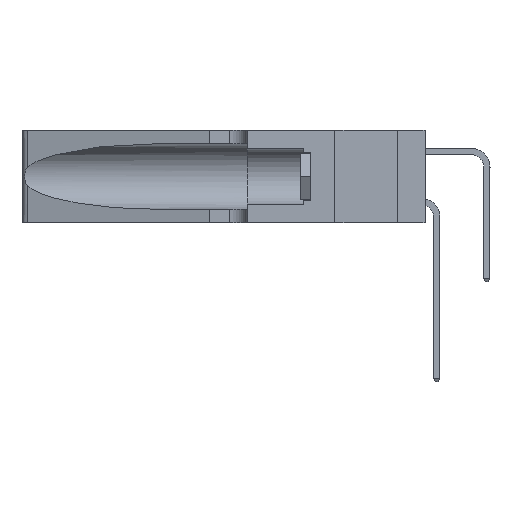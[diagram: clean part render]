
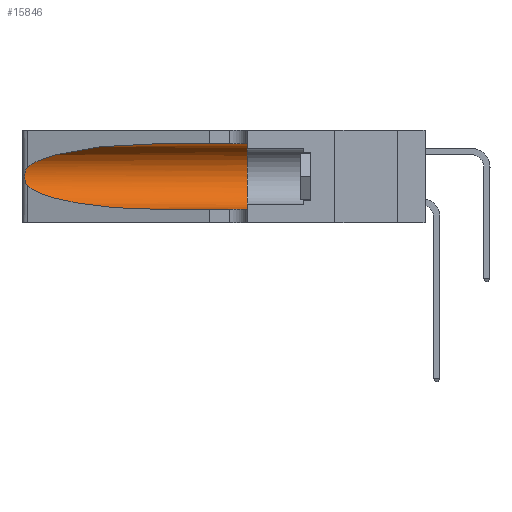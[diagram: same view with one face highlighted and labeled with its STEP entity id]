
A CAD part, left-side view. The second image highlights one B-rep face of the part: STEP entity #15846.
In plain terms, the highlighted cylindrical face has radius 3.308 mm (diameter 6.617 mm), a partial arc.
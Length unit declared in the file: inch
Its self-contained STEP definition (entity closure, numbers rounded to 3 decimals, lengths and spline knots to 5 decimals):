
#93 = CARTESIAN_POINT ( 'NONE',  ( 0.25487, 1.22718, 0.22369 ) ) ;
#305 = VERTEX_POINT ( 'NONE', #9422 ) ;
#831 = DIRECTION ( 'NONE',  ( 0., 1., 0. ) ) ;
#888 = ORIENTED_EDGE ( 'NONE', *, *, #11767, .T. ) ;
#2963 = DIRECTION ( 'NONE',  ( 0., -1., 0. ) ) ;
#3109 = CARTESIAN_POINT ( 'NONE',  ( 0.25487, 1.22718, 0.14631 ) ) ;
#3150 = FACE_OUTER_BOUND ( 'NONE', #14879, .T. ) ;
#3335 = VERTEX_POINT ( 'NONE', #10628 ) ;
#3477 = LINE ( 'NONE', #27125, #15596 ) ;
#3685 = CARTESIAN_POINT ( 'NONE',  ( 0.1305, 1.61858, 0.31525 ) ) ;
#3847 = CARTESIAN_POINT ( 'NONE',  ( 0.26018, 1.23835, 0.19895 ) ) ;
#4700 = DIRECTION ( 'NONE',  ( 0., 0., 1. ) ) ;
#5133 = AXIS2_PLACEMENT_3D ( 'NONE', #23783, #2963, #23971 ) ;
#5349 = VERTEX_POINT ( 'NONE', #10563 ) ;
#5922 = CARTESIAN_POINT ( 'NONE',  ( 0.25555, 1.22994, 0.2215 ) ) ;
#6010 = CARTESIAN_POINT ( 'NONE',  ( 0.25787, 1.23484, 0.2124 ) ) ;
#6208 = EDGE_CURVE ( 'NONE', #305, #3335, #11257, .T. ) ;
#6862 = ORIENTED_EDGE ( 'NONE', *, *, #12473, .F. ) ;
#7387 = CARTESIAN_POINT ( 'NONE',  ( 0.18966, 0.96281, 0.05475 ) ) ;
#8025 = CARTESIAN_POINT ( 'NONE',  ( 0.25856, 1.23593, 0.16098 ) ) ;
#8191 = CARTESIAN_POINT ( 'NONE',  ( 0.18966, 0.96281, 0.31525 ) ) ;
#8220 = LINE ( 'NONE', #3685, #18137 ) ;
#8479 = VERTEX_POINT ( 'NONE', #10007 ) ;
#9422 = CARTESIAN_POINT ( 'NONE',  ( 0.1305, 0.72297, 0.31525 ) ) ;
#10007 = CARTESIAN_POINT ( 'NONE',  ( 0.25487, 1.22718, 0.14631 ) ) ;
#10128 = CARTESIAN_POINT ( 'NONE',  ( 0.25639, 1.23186, 0.15144 ) ) ;
#10563 = CARTESIAN_POINT ( 'NONE',  ( 0.1305, 0.35, 0.31525 ) ) ;
#10628 = CARTESIAN_POINT ( 'NONE',  ( 0.25487, 1.22718, 0.22369 ) ) ;
#11150 = ORIENTED_EDGE ( 'NONE', *, *, #6208, .T. ) ;
#11257 =( BOUNDED_CURVE ( )  B_SPLINE_CURVE ( 3, ( #23757, #8191, #18303, #93 ),
 .UNSPECIFIED., .F., .T. ) 
 B_SPLINE_CURVE_WITH_KNOTS ( ( 4, 4 ),
 ( 1.5708, 2.84003 ),
 .UNSPECIFIED. ) 
 CURVE ( )  GEOMETRIC_REPRESENTATION_ITEM ( )  RATIONAL_B_SPLINE_CURVE ( ( 1., 0.87, 0.87, 1. ) ) 
 REPRESENTATION_ITEM ( '' )  );
#11392 = VERTEX_POINT ( 'NONE', #21391 ) ;
#11767 = EDGE_CURVE ( 'NONE', #8479, #15168, #16161, .T. ) ;
#12261 = CARTESIAN_POINT ( 'NONE',  ( 0.25789, 1.23486, 0.15765 ) ) ;
#12436 = CARTESIAN_POINT ( 'NONE',  ( 0.25854, 1.2359, 0.20912 ) ) ;
#12473 = EDGE_CURVE ( 'NONE', #305, #5349, #8220, .T. ) ;
#13924 = CARTESIAN_POINT ( 'NONE',  ( 0.1305, 0.72297, 0.05475 ) ) ;
#14403 = CARTESIAN_POINT ( 'NONE',  ( 0.26075, 1.23896, 0.178 ) ) ;
#14557 = DIRECTION ( 'NONE',  ( 0., -1., 0. ) ) ;
#14879 = EDGE_LOOP ( 'NONE', ( #11150, #17002, #888, #19067, #15684, #6862 ) ) ;
#14998 = CARTESIAN_POINT ( 'NONE',  ( 0.1305, 0.72297, 0.05475 ) ) ;
#15168 = VERTEX_POINT ( 'NONE', #14998 ) ;
#15449 = EDGE_CURVE ( 'NONE', #5349, #11392, #24511, .T. ) ;
#15596 = VECTOR ( 'NONE', #14557, 39.37008 ) ;
#15684 = ORIENTED_EDGE ( 'NONE', *, *, #15449, .F. ) ;
#15846 = ADVANCED_FACE ( 'NONE', ( #3150 ), #19951, .F. ) ;
#16161 =( BOUNDED_CURVE ( )  B_SPLINE_CURVE ( 3, ( #3109, #20224, #7387, #13924 ),
 .UNSPECIFIED., .F., .F. ) 
 B_SPLINE_CURVE_WITH_KNOTS ( ( 4, 4 ),
 ( 3.44316, 4.71239 ),
 .UNSPECIFIED. ) 
 CURVE ( )  GEOMETRIC_REPRESENTATION_ITEM ( )  RATIONAL_B_SPLINE_CURVE ( ( 1., 0.87, 0.87, 1. ) ) 
 REPRESENTATION_ITEM ( '' )  );
#17002 = ORIENTED_EDGE ( 'NONE', *, *, #21338, .T. ) ;
#17110 = EDGE_CURVE ( 'NONE', #15168, #11392, #3477, .T. ) ;
#18137 = VECTOR ( 'NONE', #18405, 39.37008 ) ;
#18303 = CARTESIAN_POINT ( 'NONE',  ( 0.2373, 1.15595, 0.28018 ) ) ;
#18405 = DIRECTION ( 'NONE',  ( 0., -1., 0. ) ) ;
#18470 = CARTESIAN_POINT ( 'NONE',  ( 0.25487, 1.22718, 0.22369 ) ) ;
#18564 = CARTESIAN_POINT ( 'NONE',  ( 0.26075, 1.23896, 0.19203 ) ) ;
#18832 = CARTESIAN_POINT ( 'NONE',  ( 0.25555, 1.22993, 0.14849 ) ) ;
#18867 = B_SPLINE_CURVE_WITH_KNOTS ( 'NONE', 3,
 ( #18470, #5922, #20692, #6010, #12436, #3847, #18564, #14403, #20769, #8025, #12261, #10128, #18832, #25108 ),
 .UNSPECIFIED., .F., .F.,
 ( 4, 2, 2, 2, 2, 2, 4 ),
 ( 0., 0.00027, 0.00053, 0.00107, 0.0016, 0.00187, 0.00214 ),
 .UNSPECIFIED. ) ;
#19067 = ORIENTED_EDGE ( 'NONE', *, *, #17110, .T. ) ;
#19951 = CYLINDRICAL_SURFACE ( 'NONE', #5133, 0.13025 ) ;
#20224 = CARTESIAN_POINT ( 'NONE',  ( 0.2373, 1.15595, 0.08982 ) ) ;
#20692 = CARTESIAN_POINT ( 'NONE',  ( 0.25639, 1.23184, 0.21858 ) ) ;
#20769 = CARTESIAN_POINT ( 'NONE',  ( 0.26017, 1.23833, 0.17102 ) ) ;
#21338 = EDGE_CURVE ( 'NONE', #3335, #8479, #18867, .T. ) ;
#21391 = CARTESIAN_POINT ( 'NONE',  ( 0.1305, 0.35, 0.05475 ) ) ;
#23638 = CARTESIAN_POINT ( 'NONE',  ( 0.1305, 0.35, 0.185 ) ) ;
#23757 = CARTESIAN_POINT ( 'NONE',  ( 0.1305, 0.72297, 0.31525 ) ) ;
#23783 = CARTESIAN_POINT ( 'NONE',  ( 0.1305, 1.61858, 0.185 ) ) ;
#23971 = DIRECTION ( 'NONE',  ( 0., 0., -1. ) ) ;
#24511 = CIRCLE ( 'NONE', #25511, 0.13025 ) ;
#25108 = CARTESIAN_POINT ( 'NONE',  ( 0.25487, 1.22718, 0.14631 ) ) ;
#25511 = AXIS2_PLACEMENT_3D ( 'NONE', #23638, #831, #4700 ) ;
#27125 = CARTESIAN_POINT ( 'NONE',  ( 0.1305, 1.61858, 0.05475 ) ) ;
